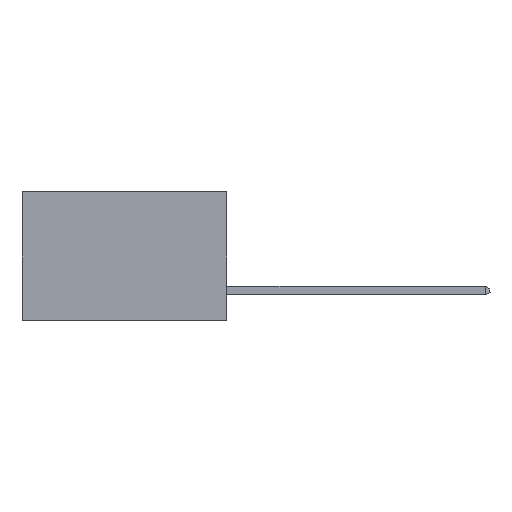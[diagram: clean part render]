
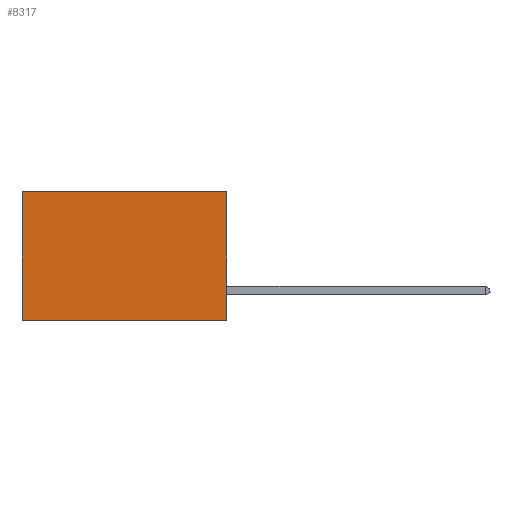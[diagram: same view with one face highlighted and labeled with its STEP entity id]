
A CAD part, left-side view. The second image highlights one B-rep face of the part: STEP entity #8317.
In plain terms, the highlighted planar face has unit normal (-1, 0, 0).
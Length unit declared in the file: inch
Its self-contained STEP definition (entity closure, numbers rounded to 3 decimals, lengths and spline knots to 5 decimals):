
#1753 = ORIENTED_EDGE ( 'NONE', *, *, #20402, .F. ) ;
#2649 = FACE_OUTER_BOUND ( 'NONE', #23718, .T. ) ;
#2673 = EDGE_CURVE ( 'NONE', #22444, #20138, #11020, .T. ) ;
#3154 = EDGE_CURVE ( 'NONE', #22444, #13006, #7689, .T. ) ;
#3369 = VECTOR ( 'NONE', #9611, 39.37008 ) ;
#5351 = CARTESIAN_POINT ( 'NONE',  ( 0.277, 0.59, -0.37 ) ) ;
#7689 = LINE ( 'NONE', #13899, #23993 ) ;
#8317 = ADVANCED_FACE ( 'NONE', ( #2649 ), #16104, .F. ) ;
#9047 = ORIENTED_EDGE ( 'NONE', *, *, #2673, .T. ) ;
#9355 = DIRECTION ( 'NONE',  ( 0., 1., 0. ) ) ;
#9611 = DIRECTION ( 'NONE',  ( 0., 0., -1. ) ) ;
#10882 = LINE ( 'NONE', #12242, #21730 ) ;
#11020 = LINE ( 'NONE', #15905, #21242 ) ;
#12211 = VERTEX_POINT ( 'NONE', #20991 ) ;
#12242 = CARTESIAN_POINT ( 'NONE',  ( 0.277, 0., -0.37 ) ) ;
#13006 = VERTEX_POINT ( 'NONE', #25537 ) ;
#13899 = CARTESIAN_POINT ( 'NONE',  ( 0.277, 0., -0.37 ) ) ;
#14401 = EDGE_CURVE ( 'NONE', #20138, #12211, #25184, .T. ) ;
#14493 = DIRECTION ( 'NONE',  ( 0., 0., -1. ) ) ;
#14811 = AXIS2_PLACEMENT_3D ( 'NONE', #16018, #16012, #15987 ) ;
#15905 = CARTESIAN_POINT ( 'NONE',  ( 0.277, 0., 0. ) ) ;
#15987 = DIRECTION ( 'NONE',  ( 0., 0., -1. ) ) ;
#16012 = DIRECTION ( 'NONE',  ( 1., 0., 0. ) ) ;
#16018 = CARTESIAN_POINT ( 'NONE',  ( 0.277, 0., -0.37 ) ) ;
#16104 = PLANE ( 'NONE',  #14811 ) ;
#17541 = CARTESIAN_POINT ( 'NONE',  ( 0.277, 0.59, 0. ) ) ;
#19319 = CARTESIAN_POINT ( 'NONE',  ( 0.277, 0., 0. ) ) ;
#20138 = VERTEX_POINT ( 'NONE', #17541 ) ;
#20402 = EDGE_CURVE ( 'NONE', #13006, #12211, #10882, .T. ) ;
#20991 = CARTESIAN_POINT ( 'NONE',  ( 0.277, 0.59, -0.37 ) ) ;
#21242 = VECTOR ( 'NONE', #9355, 39.37008 ) ;
#21730 = VECTOR ( 'NONE', #26299, 39.37008 ) ;
#22444 = VERTEX_POINT ( 'NONE', #19319 ) ;
#23718 = EDGE_LOOP ( 'NONE', ( #25106, #1753, #25857, #9047 ) ) ;
#23993 = VECTOR ( 'NONE', #14493, 39.37008 ) ;
#25106 = ORIENTED_EDGE ( 'NONE', *, *, #14401, .T. ) ;
#25184 = LINE ( 'NONE', #5351, #3369 ) ;
#25537 = CARTESIAN_POINT ( 'NONE',  ( 0.277, 0., -0.37 ) ) ;
#25857 = ORIENTED_EDGE ( 'NONE', *, *, #3154, .F. ) ;
#26299 = DIRECTION ( 'NONE',  ( 0., 1., 0. ) ) ;
